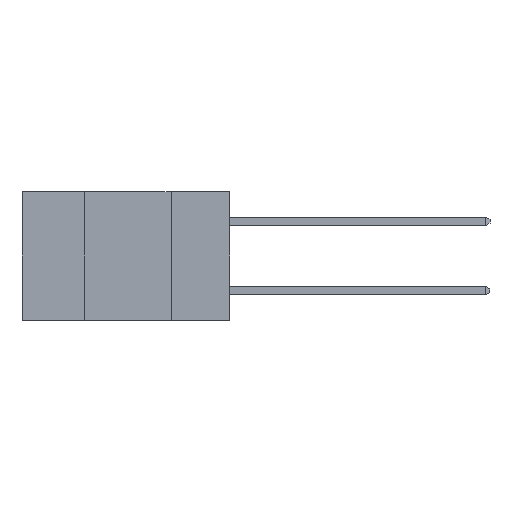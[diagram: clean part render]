
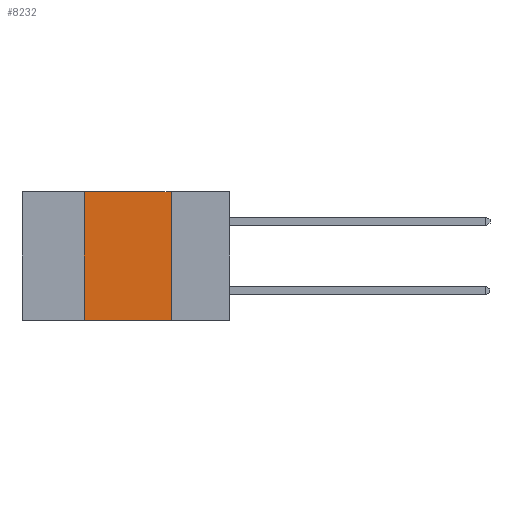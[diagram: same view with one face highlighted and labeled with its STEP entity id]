
A CAD part, left-side view. The second image highlights one B-rep face of the part: STEP entity #8232.
In plain terms, the highlighted planar face has unit normal (-1, 0, 0).
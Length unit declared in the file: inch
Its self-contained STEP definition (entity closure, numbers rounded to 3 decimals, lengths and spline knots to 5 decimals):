
#611 = VECTOR ( 'NONE', #4726, 39.37008 ) ;
#682 = CARTESIAN_POINT ( 'NONE',  ( 0., 0.6, 0. ) ) ;
#722 = AXIS2_PLACEMENT_3D ( 'NONE', #8628, #3285, #3097 ) ;
#1099 = CARTESIAN_POINT ( 'NONE',  ( 0., 0.42, -0.37 ) ) ;
#1151 = CARTESIAN_POINT ( 'NONE',  ( 0., 0.42, 0. ) ) ;
#1505 = CARTESIAN_POINT ( 'NONE',  ( 0., 0.6, -0.37 ) ) ;
#2213 = VERTEX_POINT ( 'NONE', #7421 ) ;
#2346 = CARTESIAN_POINT ( 'NONE',  ( 0., 0.17, 0. ) ) ;
#2776 = LINE ( 'NONE', #2346, #611 ) ;
#3097 = DIRECTION ( 'NONE',  ( 0., 0., -1. ) ) ;
#3285 = DIRECTION ( 'NONE',  ( 1., 0., 0. ) ) ;
#3395 = PLANE ( 'NONE',  #722 ) ;
#3855 = EDGE_CURVE ( 'NONE', #2213, #8875, #2776, .T. ) ;
#4337 = ORIENTED_EDGE ( 'NONE', *, *, #5577, .F. ) ;
#4437 = LINE ( 'NONE', #682, #9947 ) ;
#4450 = ORIENTED_EDGE ( 'NONE', *, *, #3855, .F. ) ;
#4726 = DIRECTION ( 'NONE',  ( 0., 0., -1. ) ) ;
#4865 = FACE_OUTER_BOUND ( 'NONE', #8143, .T. ) ;
#5015 = LINE ( 'NONE', #1505, #8795 ) ;
#5271 = CARTESIAN_POINT ( 'NONE',  ( 0., 0.42, 0. ) ) ;
#5577 = EDGE_CURVE ( 'NONE', #9265, #2213, #4437, .T. ) ;
#6431 = DIRECTION ( 'NONE',  ( 0., -1., 0. ) ) ;
#6666 = VERTEX_POINT ( 'NONE', #1099 ) ;
#6724 = EDGE_CURVE ( 'NONE', #6666, #8875, #5015, .T. ) ;
#7110 = CARTESIAN_POINT ( 'NONE',  ( 0., 0.17, -0.37 ) ) ;
#7246 = DIRECTION ( 'NONE',  ( 0., 0., 1. ) ) ;
#7360 = LINE ( 'NONE', #5271, #9554 ) ;
#7421 = CARTESIAN_POINT ( 'NONE',  ( 0., 0.17, 0. ) ) ;
#7781 = ORIENTED_EDGE ( 'NONE', *, *, #8189, .F. ) ;
#8143 = EDGE_LOOP ( 'NONE', ( #4450, #4337, #7781, #8951 ) ) ;
#8189 = EDGE_CURVE ( 'NONE', #6666, #9265, #7360, .T. ) ;
#8232 = ADVANCED_FACE ( 'NONE', ( #4865 ), #3395, .F. ) ;
#8628 = CARTESIAN_POINT ( 'NONE',  ( 0., 0.6, 0. ) ) ;
#8795 = VECTOR ( 'NONE', #6431, 39.37008 ) ;
#8875 = VERTEX_POINT ( 'NONE', #7110 ) ;
#8942 = DIRECTION ( 'NONE',  ( 0., -1., 0. ) ) ;
#8951 = ORIENTED_EDGE ( 'NONE', *, *, #6724, .T. ) ;
#9265 = VERTEX_POINT ( 'NONE', #1151 ) ;
#9554 = VECTOR ( 'NONE', #7246, 39.37008 ) ;
#9947 = VECTOR ( 'NONE', #8942, 39.37008 ) ;
